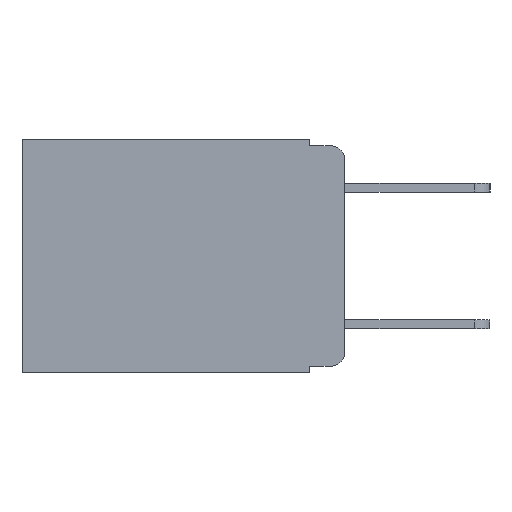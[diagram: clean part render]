
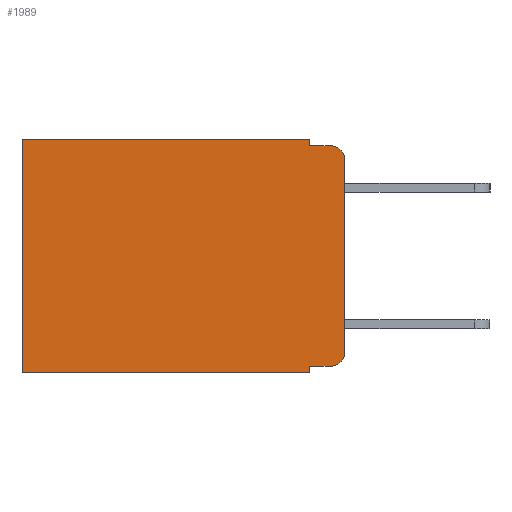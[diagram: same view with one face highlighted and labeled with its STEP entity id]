
A CAD part, left-side view. The second image highlights one B-rep face of the part: STEP entity #1989.
In plain terms, the highlighted planar face has unit normal (-1, 0, 0).
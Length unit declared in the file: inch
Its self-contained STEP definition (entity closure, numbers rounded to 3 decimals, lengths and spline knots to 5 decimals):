
#588 = CARTESIAN_POINT ( 'NONE',  ( 0.298, 0.473, 0. ) ) ;
#1059 = VERTEX_POINT ( 'NONE', #8483 ) ;
#1393 = LINE ( 'NONE', #14352, #9942 ) ;
#1989 = ADVANCED_FACE ( 'NONE', ( #6797 ), #18513, .F. ) ;
#2405 = EDGE_CURVE ( 'NONE', #15409, #12385, #18433, .T. ) ;
#2492 = DIRECTION ( 'NONE',  ( 0., 0., -1. ) ) ;
#2662 = CARTESIAN_POINT ( 'NONE',  ( 0.298, 0.051, 0. ) ) ;
#2850 = EDGE_CURVE ( 'NONE', #4657, #14928, #7770, .T. ) ;
#3122 = LINE ( 'NONE', #7167, #10884 ) ;
#3137 = EDGE_CURVE ( 'NONE', #11903, #12968, #8726, .T. ) ;
#3144 = EDGE_CURVE ( 'NONE', #11903, #16406, #15882, .T. ) ;
#3167 = EDGE_CURVE ( 'NONE', #1059, #16406, #7732, .T. ) ;
#3172 = EDGE_CURVE ( 'NONE', #15409, #1059, #15064, .T. ) ;
#3177 = EDGE_CURVE ( 'NONE', #12385, #14928, #3122, .T. ) ;
#3202 = EDGE_CURVE ( 'NONE', #15645, #4657, #17321, .T. ) ;
#3204 = EDGE_CURVE ( 'NONE', #15645, #3846, #1393, .T. ) ;
#3205 = EDGE_CURVE ( 'NONE', #3846, #12968, #13827, .T. ) ;
#3607 = CARTESIAN_POINT ( 'NONE',  ( 0.298, 0.473, -0.343 ) ) ;
#3846 = VERTEX_POINT ( 'NONE', #15287 ) ;
#4303 = ORIENTED_EDGE ( 'NONE', *, *, #2850, .F. ) ;
#4657 = VERTEX_POINT ( 'NONE', #11066 ) ;
#4990 = CARTESIAN_POINT ( 'NONE',  ( 0.298, 0., -0.03 ) ) ;
#5545 = AXIS2_PLACEMENT_3D ( 'NONE', #7757, #7616, #12904 ) ;
#5966 = ORIENTED_EDGE ( 'NONE', *, *, #3202, .F. ) ;
#6104 = CARTESIAN_POINT ( 'NONE',  ( 0.298, 0.051, 0. ) ) ;
#6218 = ORIENTED_EDGE ( 'NONE', *, *, #3205, .T. ) ;
#6707 = DIRECTION ( 'NONE',  ( -1., 0., 0. ) ) ;
#6797 = FACE_OUTER_BOUND ( 'NONE', #13076, .T. ) ;
#6806 = CARTESIAN_POINT ( 'NONE',  ( 0.298, 0.02, -0.313 ) ) ;
#7167 = CARTESIAN_POINT ( 'NONE',  ( 0.298, 0.473, 0. ) ) ;
#7479 = DIRECTION ( 'NONE',  ( 0., 0., -1. ) ) ;
#7616 = DIRECTION ( 'NONE',  ( -1., 0., 0. ) ) ;
#7732 = LINE ( 'NONE', #15089, #18571 ) ;
#7757 = CARTESIAN_POINT ( 'NONE',  ( 0.298, 0.02, -0.03 ) ) ;
#7770 = LINE ( 'NONE', #10816, #15097 ) ;
#8101 = DIRECTION ( 'NONE',  ( 0., 0., -1. ) ) ;
#8276 = DIRECTION ( 'NONE',  ( 0., 1., 0. ) ) ;
#8302 = CARTESIAN_POINT ( 'NONE',  ( 0.298, 0.051, 0. ) ) ;
#8483 = CARTESIAN_POINT ( 'NONE',  ( 0.298, 0.051, -0.01 ) ) ;
#8726 = LINE ( 'NONE', #18813, #12235 ) ;
#9184 = DIRECTION ( 'NONE',  ( 0., -1., 0. ) ) ;
#9351 = ORIENTED_EDGE ( 'NONE', *, *, #3204, .T. ) ;
#9922 = ORIENTED_EDGE ( 'NONE', *, *, #3137, .F. ) ;
#9942 = VECTOR ( 'NONE', #14998, 39.37008 ) ;
#10660 = DIRECTION ( 'NONE',  ( 0., 1., 0. ) ) ;
#10816 = CARTESIAN_POINT ( 'NONE',  ( 0.298, 0., -0.343 ) ) ;
#10884 = VECTOR ( 'NONE', #14697, 39.37008 ) ;
#11066 = CARTESIAN_POINT ( 'NONE',  ( 0.298, 0.051, -0.343 ) ) ;
#11351 = VECTOR ( 'NONE', #2492, 39.37008 ) ;
#11700 = CARTESIAN_POINT ( 'NONE',  ( 0.298, 0., 0. ) ) ;
#11771 = ORIENTED_EDGE ( 'NONE', *, *, #3144, .T. ) ;
#11903 = VERTEX_POINT ( 'NONE', #4990 ) ;
#12235 = VECTOR ( 'NONE', #8101, 39.37008 ) ;
#12385 = VERTEX_POINT ( 'NONE', #588 ) ;
#12464 = DIRECTION ( 'NONE',  ( 0., 0., -1. ) ) ;
#12904 = DIRECTION ( 'NONE',  ( 0., 0., -1. ) ) ;
#12948 = ORIENTED_EDGE ( 'NONE', *, *, #3167, .F. ) ;
#12968 = VERTEX_POINT ( 'NONE', #17569 ) ;
#13076 = EDGE_LOOP ( 'NONE', ( #9922, #11771, #12948, #13212, #13668, #15655, #4303, #5966, #9351, #6218 ) ) ;
#13212 = ORIENTED_EDGE ( 'NONE', *, *, #3172, .F. ) ;
#13668 = ORIENTED_EDGE ( 'NONE', *, *, #2405, .T. ) ;
#13827 = CIRCLE ( 'NONE', #17373, 0.02 ) ;
#14352 = CARTESIAN_POINT ( 'NONE',  ( 0.298, 0.051, -0.333 ) ) ;
#14697 = DIRECTION ( 'NONE',  ( 0., 0., -1. ) ) ;
#14928 = VERTEX_POINT ( 'NONE', #3607 ) ;
#14998 = DIRECTION ( 'NONE',  ( 0., -1., 0. ) ) ;
#15064 = LINE ( 'NONE', #2662, #11351 ) ;
#15089 = CARTESIAN_POINT ( 'NONE',  ( 0.298, 0.051, -0.01 ) ) ;
#15097 = VECTOR ( 'NONE', #10660, 39.37008 ) ;
#15287 = CARTESIAN_POINT ( 'NONE',  ( 0.298, 0.02, -0.333 ) ) ;
#15409 = VERTEX_POINT ( 'NONE', #6104 ) ;
#15645 = VERTEX_POINT ( 'NONE', #16585 ) ;
#15655 = ORIENTED_EDGE ( 'NONE', *, *, #3177, .T. ) ;
#15688 = AXIS2_PLACEMENT_3D ( 'NONE', #18562, #18710, #18697 ) ;
#15882 = CIRCLE ( 'NONE', #5545, 0.02 ) ;
#16396 = CARTESIAN_POINT ( 'NONE',  ( 0.298, 0.02, -0.01 ) ) ;
#16406 = VERTEX_POINT ( 'NONE', #16396 ) ;
#16585 = CARTESIAN_POINT ( 'NONE',  ( 0.298, 0.051, -0.333 ) ) ;
#17321 = LINE ( 'NONE', #8302, #18169 ) ;
#17373 = AXIS2_PLACEMENT_3D ( 'NONE', #6806, #6707, #7479 ) ;
#17569 = CARTESIAN_POINT ( 'NONE',  ( 0.298, 0., -0.313 ) ) ;
#18169 = VECTOR ( 'NONE', #12464, 39.37008 ) ;
#18433 = LINE ( 'NONE', #11700, #18808 ) ;
#18513 = PLANE ( 'NONE',  #15688 ) ;
#18562 = CARTESIAN_POINT ( 'NONE',  ( 0.298, 0., 0. ) ) ;
#18571 = VECTOR ( 'NONE', #9184, 39.37008 ) ;
#18697 = DIRECTION ( 'NONE',  ( 0., 0., -1. ) ) ;
#18710 = DIRECTION ( 'NONE',  ( 1., 0., 0. ) ) ;
#18808 = VECTOR ( 'NONE', #8276, 39.37008 ) ;
#18813 = CARTESIAN_POINT ( 'NONE',  ( 0.298, 0., 0. ) ) ;
